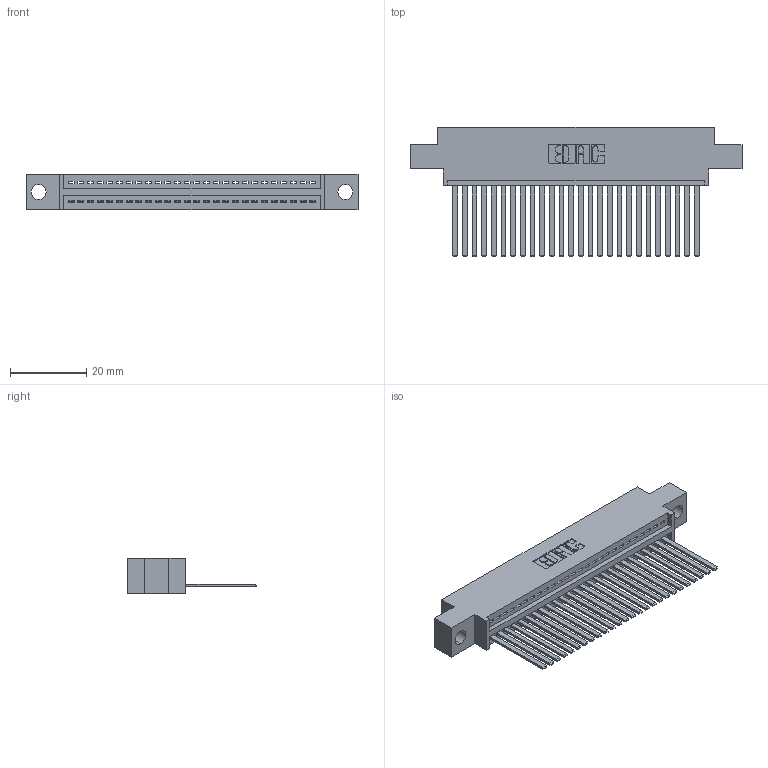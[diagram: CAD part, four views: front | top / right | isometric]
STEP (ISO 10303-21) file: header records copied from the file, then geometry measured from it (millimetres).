
FILE_DESCRIPTION (( 'STEP AP203' ), '1' );
FILE_NAME ('345-026-544-604.STEP', '2021-05-26T14:32:08', ( '' ), ( '' ), 'SwSTEP 2.0', 'SolidWorks 2020', '' );
FILE_SCHEMA (( 'CONFIG_CONTROL_DESIGN' ));
Length unit declared in the file: inch
Products named in the file (3): 345-292-001_345-293-144; 345 Part_0.170 Offset - 0.156 Dia-TI; 345-026-544-604
Assembly tree (27 placements, depth 2):
  345-026-544-604
    345 Part_0.170 Offset - 0.156 Dia-TI
    345-292-001_345-293-144  x26
Bounding box: 87.25 x 33.96 x 9.4 mm (x, y, z)
Volume: 8237.7 mm3; surface area: 11602.7 mm2
Topology: 27 solids, 27 shells, 1496 faces, 4497 edges, 2962 vertices
Faces by surface type: plane 1034, cylinder 462
Entity records: 22089 total; most frequent: CARTESIAN_POINT 3836, ORIENTED_EDGE 3794, DIRECTION 3369, EDGE_CURVE 1897, VECTOR 1665, LINE 1665, VERTEX_POINT 1262, AXIS2_PLACEMENT_3D 852
